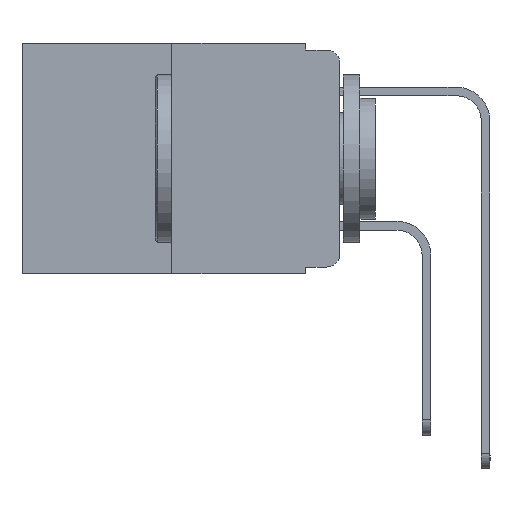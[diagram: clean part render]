
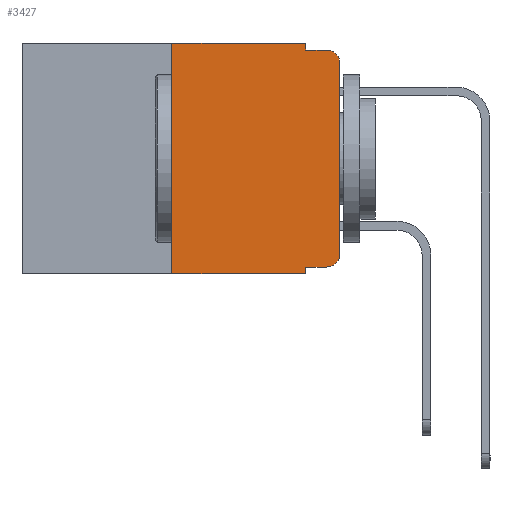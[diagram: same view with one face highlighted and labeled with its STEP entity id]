
A CAD part, left-side view. The second image highlights one B-rep face of the part: STEP entity #3427.
In plain terms, the highlighted planar face has unit normal (-1, 0, 0).
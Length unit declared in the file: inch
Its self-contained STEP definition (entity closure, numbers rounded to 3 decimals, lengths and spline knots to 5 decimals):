
#492 = DIRECTION ( 'NONE',  ( 0., 0., 1. ) ) ;
#582 = VERTEX_POINT ( 'NONE', #3348 ) ;
#801 = CARTESIAN_POINT ( 'NONE',  ( 0., 0.051, -0.333 ) ) ;
#1021 = AXIS2_PLACEMENT_3D ( 'NONE', #12262, #19692, #2489 ) ;
#1086 = DIRECTION ( 'NONE',  ( 0., 0., 1. ) ) ;
#1128 = EDGE_CURVE ( 'NONE', #4817, #10208, #2039, .T. ) ;
#1137 = VECTOR ( 'NONE', #17697, 39.37008 ) ;
#1325 = ORIENTED_EDGE ( 'NONE', *, *, #3578, .F. ) ;
#1517 = CARTESIAN_POINT ( 'NONE',  ( 0., 0.02, -0.313 ) ) ;
#1548 = AXIS2_PLACEMENT_3D ( 'NONE', #1517, #22360, #17055 ) ;
#1625 = EDGE_CURVE ( 'NONE', #19464, #13480, #6486, .T. ) ;
#1764 = VERTEX_POINT ( 'NONE', #14574 ) ;
#1999 = EDGE_LOOP ( 'NONE', ( #23954, #15845, #16292, #12402, #20933, #19542, #2513, #1325, #17361, #4404 ) ) ;
#2039 = LINE ( 'NONE', #6023, #11032 ) ;
#2489 = DIRECTION ( 'NONE',  ( 0., 0., -1. ) ) ;
#2513 = ORIENTED_EDGE ( 'NONE', *, *, #23077, .T. ) ;
#3038 = VECTOR ( 'NONE', #19477, 39.37008 ) ;
#3348 = CARTESIAN_POINT ( 'NONE',  ( 0., 0.051, 0. ) ) ;
#3427 = ADVANCED_FACE ( 'NONE', ( #12130 ), #4408, .F. ) ;
#3473 = VECTOR ( 'NONE', #14670, 39.37008 ) ;
#3570 = VECTOR ( 'NONE', #492, 39.37008 ) ;
#3578 = EDGE_CURVE ( 'NONE', #19464, #9537, #18400, .T. ) ;
#4303 = EDGE_CURVE ( 'NONE', #10208, #582, #20013, .T. ) ;
#4404 = ORIENTED_EDGE ( 'NONE', *, *, #13238, .T. ) ;
#4408 = PLANE ( 'NONE',  #1021 ) ;
#4785 = CARTESIAN_POINT ( 'NONE',  ( 0., 0.02, -0.03 ) ) ;
#4817 = VERTEX_POINT ( 'NONE', #16343 ) ;
#5110 = LINE ( 'NONE', #22925, #21090 ) ;
#5984 = DIRECTION ( 'NONE',  ( 0., -1., 0. ) ) ;
#6023 = CARTESIAN_POINT ( 'NONE',  ( 0., 0.25, 0. ) ) ;
#6263 = VERTEX_POINT ( 'NONE', #18886 ) ;
#6486 = LINE ( 'NONE', #12290, #6967 ) ;
#6703 = VECTOR ( 'NONE', #11952, 39.37008 ) ;
#6967 = VECTOR ( 'NONE', #5984, 39.37008 ) ;
#7804 = CARTESIAN_POINT ( 'NONE',  ( 0., 0.473, 0. ) ) ;
#8571 = CARTESIAN_POINT ( 'NONE',  ( 0., 0., 0. ) ) ;
#8629 = VERTEX_POINT ( 'NONE', #15989 ) ;
#9537 = VERTEX_POINT ( 'NONE', #11706 ) ;
#10127 = LINE ( 'NONE', #13749, #6703 ) ;
#10208 = VERTEX_POINT ( 'NONE', #17617 ) ;
#11032 = VECTOR ( 'NONE', #1086, 39.37008 ) ;
#11262 = EDGE_CURVE ( 'NONE', #1764, #6263, #23203, .T. ) ;
#11518 = DIRECTION ( 'NONE',  ( 0., -1., 0. ) ) ;
#11706 = CARTESIAN_POINT ( 'NONE',  ( 0., 0.051, -0.343 ) ) ;
#11952 = DIRECTION ( 'NONE',  ( 0., 0., -1. ) ) ;
#12130 = FACE_OUTER_BOUND ( 'NONE', #1999, .T. ) ;
#12172 = EDGE_CURVE ( 'NONE', #24090, #1764, #22165, .T. ) ;
#12252 = DIRECTION ( 'NONE',  ( 0., 0., -1. ) ) ;
#12262 = CARTESIAN_POINT ( 'NONE',  ( 0., 0.473, 0. ) ) ;
#12290 = CARTESIAN_POINT ( 'NONE',  ( 0., 0.051, -0.333 ) ) ;
#12380 = DIRECTION ( 'NONE',  ( -1., 0., 0. ) ) ;
#12402 = ORIENTED_EDGE ( 'NONE', *, *, #22769, .F. ) ;
#12653 = CIRCLE ( 'NONE', #1548, 0.02 ) ;
#13238 = EDGE_CURVE ( 'NONE', #13480, #24090, #12653, .T. ) ;
#13480 = VERTEX_POINT ( 'NONE', #18085 ) ;
#13749 = CARTESIAN_POINT ( 'NONE',  ( 0., 0.051, 0. ) ) ;
#14574 = CARTESIAN_POINT ( 'NONE',  ( 0., 0., -0.03 ) ) ;
#14670 = DIRECTION ( 'NONE',  ( 0., 0., -1. ) ) ;
#15038 = CARTESIAN_POINT ( 'NONE',  ( 0., 0., -0.313 ) ) ;
#15109 = CARTESIAN_POINT ( 'NONE',  ( 0., 0.051, -0.01 ) ) ;
#15845 = ORIENTED_EDGE ( 'NONE', *, *, #11262, .T. ) ;
#15989 = CARTESIAN_POINT ( 'NONE',  ( 0., 0.051, -0.01 ) ) ;
#16292 = ORIENTED_EDGE ( 'NONE', *, *, #24487, .F. ) ;
#16343 = CARTESIAN_POINT ( 'NONE',  ( 0., 0.25, -0.343 ) ) ;
#17041 = LINE ( 'NONE', #15109, #3038 ) ;
#17055 = DIRECTION ( 'NONE',  ( 0., 0., -1. ) ) ;
#17361 = ORIENTED_EDGE ( 'NONE', *, *, #1625, .T. ) ;
#17617 = CARTESIAN_POINT ( 'NONE',  ( 0., 0.25, 0. ) ) ;
#17697 = DIRECTION ( 'NONE',  ( 0., -1., 0. ) ) ;
#18085 = CARTESIAN_POINT ( 'NONE',  ( 0., 0.02, -0.333 ) ) ;
#18400 = LINE ( 'NONE', #20456, #3473 ) ;
#18709 = AXIS2_PLACEMENT_3D ( 'NONE', #4785, #12380, #12252 ) ;
#18886 = CARTESIAN_POINT ( 'NONE',  ( 0., 0.02, -0.01 ) ) ;
#19464 = VERTEX_POINT ( 'NONE', #801 ) ;
#19477 = DIRECTION ( 'NONE',  ( 0., -1., 0. ) ) ;
#19542 = ORIENTED_EDGE ( 'NONE', *, *, #1128, .F. ) ;
#19692 = DIRECTION ( 'NONE',  ( 1., 0., 0. ) ) ;
#20013 = LINE ( 'NONE', #7804, #1137 ) ;
#20456 = CARTESIAN_POINT ( 'NONE',  ( 0., 0.051, 0. ) ) ;
#20933 = ORIENTED_EDGE ( 'NONE', *, *, #4303, .F. ) ;
#21090 = VECTOR ( 'NONE', #11518, 39.37008 ) ;
#22165 = LINE ( 'NONE', #8571, #3570 ) ;
#22360 = DIRECTION ( 'NONE',  ( -1., 0., 0. ) ) ;
#22769 = EDGE_CURVE ( 'NONE', #582, #8629, #10127, .T. ) ;
#22925 = CARTESIAN_POINT ( 'NONE',  ( 0., 0.473, -0.343 ) ) ;
#23077 = EDGE_CURVE ( 'NONE', #4817, #9537, #5110, .T. ) ;
#23203 = CIRCLE ( 'NONE', #18709, 0.02 ) ;
#23954 = ORIENTED_EDGE ( 'NONE', *, *, #12172, .T. ) ;
#24090 = VERTEX_POINT ( 'NONE', #15038 ) ;
#24487 = EDGE_CURVE ( 'NONE', #8629, #6263, #17041, .T. ) ;
